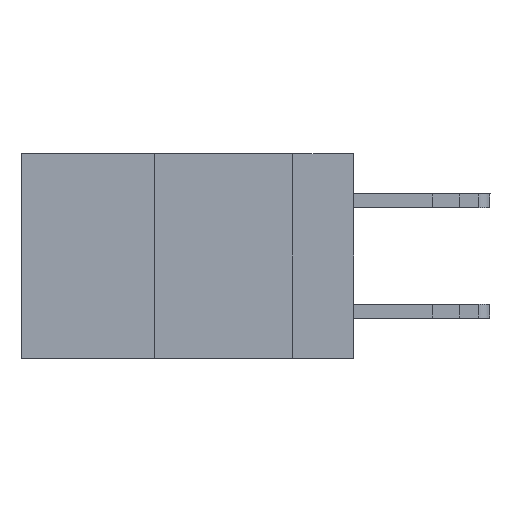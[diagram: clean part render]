
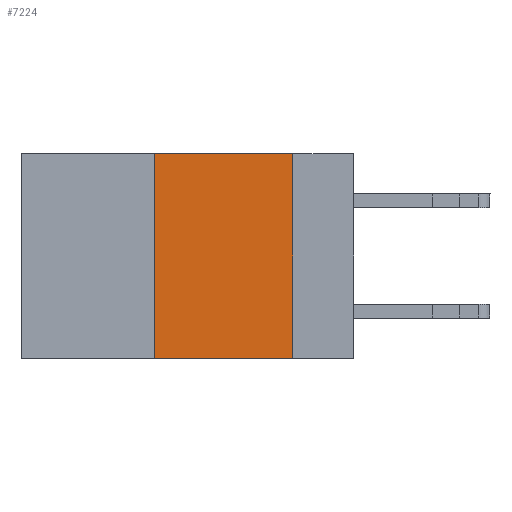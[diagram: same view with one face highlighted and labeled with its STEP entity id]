
A CAD part, left-side view. The second image highlights one B-rep face of the part: STEP entity #7224.
In plain terms, the highlighted planar face has unit normal (-1, 0, 0).
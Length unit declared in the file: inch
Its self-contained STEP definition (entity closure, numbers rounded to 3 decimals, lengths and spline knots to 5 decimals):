
#229 = ORIENTED_EDGE ( 'NONE', *, *, #7165, .F. ) ;
#559 = EDGE_LOOP ( 'NONE', ( #9330, #7349, #229, #2303 ) ) ;
#914 = VECTOR ( 'NONE', #16582, 39.37008 ) ;
#1004 = VERTEX_POINT ( 'NONE', #5278 ) ;
#1293 = VERTEX_POINT ( 'NONE', #2465 ) ;
#1649 = LINE ( 'NONE', #3515, #8590 ) ;
#1764 = CARTESIAN_POINT ( 'NONE',  ( 0., 0.11, 0. ) ) ;
#2303 = ORIENTED_EDGE ( 'NONE', *, *, #11973, .T. ) ;
#2465 = CARTESIAN_POINT ( 'NONE',  ( 0., 0.11, 0. ) ) ;
#3515 = CARTESIAN_POINT ( 'NONE',  ( 0., 0.6, 0. ) ) ;
#3643 = CARTESIAN_POINT ( 'NONE',  ( 0., 0.36, -0.37 ) ) ;
#3765 = CARTESIAN_POINT ( 'NONE',  ( 0., 0.6, -0.37 ) ) ;
#4127 = DIRECTION ( 'NONE',  ( 0., 0., -1. ) ) ;
#4161 = EDGE_CURVE ( 'NONE', #1293, #1004, #16791, .T. ) ;
#5278 = CARTESIAN_POINT ( 'NONE',  ( 0., 0.11, -0.37 ) ) ;
#6411 = VERTEX_POINT ( 'NONE', #11301 ) ;
#6762 = DIRECTION ( 'NONE',  ( 0., -1., 0. ) ) ;
#6953 = CARTESIAN_POINT ( 'NONE',  ( 0., 0.6, 0. ) ) ;
#7165 = EDGE_CURVE ( 'NONE', #13797, #6411, #13280, .T. ) ;
#7224 = ADVANCED_FACE ( 'NONE', ( #11894 ), #13015, .F. ) ;
#7335 = VECTOR ( 'NONE', #14905, 39.37008 ) ;
#7349 = ORIENTED_EDGE ( 'NONE', *, *, #11342, .F. ) ;
#8590 = VECTOR ( 'NONE', #12049, 39.37008 ) ;
#8601 = DIRECTION ( 'NONE',  ( 1., 0., 0. ) ) ;
#9330 = ORIENTED_EDGE ( 'NONE', *, *, #4161, .F. ) ;
#9929 = LINE ( 'NONE', #3765, #12406 ) ;
#11301 = CARTESIAN_POINT ( 'NONE',  ( 0., 0.36, 0. ) ) ;
#11342 = EDGE_CURVE ( 'NONE', #6411, #1293, #1649, .T. ) ;
#11894 = FACE_OUTER_BOUND ( 'NONE', #559, .T. ) ;
#11973 = EDGE_CURVE ( 'NONE', #13797, #1004, #9929, .T. ) ;
#12049 = DIRECTION ( 'NONE',  ( 0., -1., 0. ) ) ;
#12406 = VECTOR ( 'NONE', #6762, 39.37008 ) ;
#13015 = PLANE ( 'NONE',  #16680 ) ;
#13280 = LINE ( 'NONE', #13569, #914 ) ;
#13569 = CARTESIAN_POINT ( 'NONE',  ( 0., 0.36, 0. ) ) ;
#13797 = VERTEX_POINT ( 'NONE', #3643 ) ;
#14905 = DIRECTION ( 'NONE',  ( 0., 0., -1. ) ) ;
#16582 = DIRECTION ( 'NONE',  ( 0., 0., 1. ) ) ;
#16680 = AXIS2_PLACEMENT_3D ( 'NONE', #6953, #8601, #4127 ) ;
#16791 = LINE ( 'NONE', #1764, #7335 ) ;
